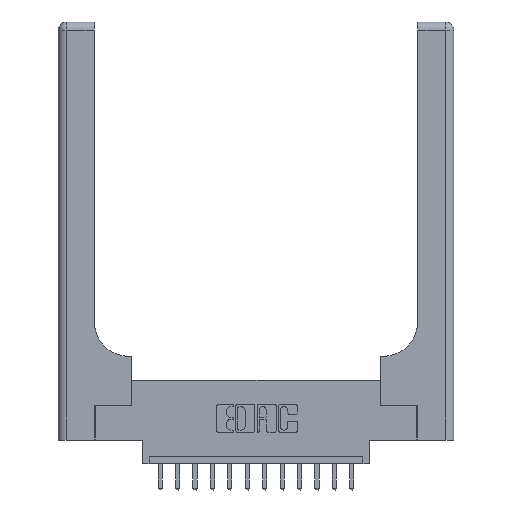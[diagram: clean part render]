
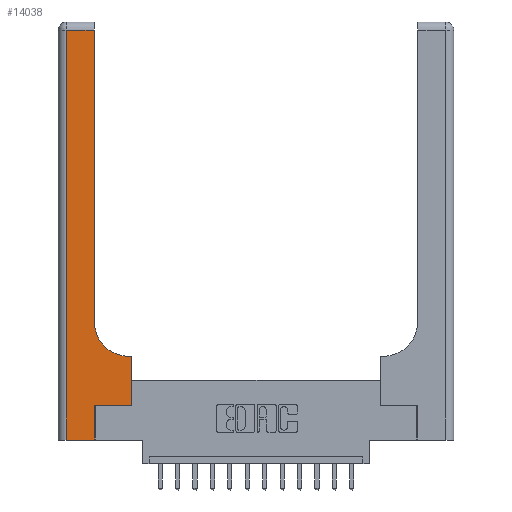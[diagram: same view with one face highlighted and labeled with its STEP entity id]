
A CAD part, top view. The second image highlights one B-rep face of the part: STEP entity #14038.
In plain terms, the highlighted planar face has unit normal (0, 0, 1).
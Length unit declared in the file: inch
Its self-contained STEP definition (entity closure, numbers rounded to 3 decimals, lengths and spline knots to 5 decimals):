
#672 = VERTEX_POINT ( 'NONE', #14484 ) ;
#717 = EDGE_LOOP ( 'NONE', ( #3443, #8007, #9765, #12176, #15172, #10499, #14028, #17084, #14723 ) ) ;
#1391 = CARTESIAN_POINT ( 'NONE',  ( 0.26, 2.94, 0.37 ) ) ;
#1451 = DIRECTION ( 'NONE',  ( 1., 0., 0. ) ) ;
#1673 = LINE ( 'NONE', #4305, #2613 ) ;
#2115 = AXIS2_PLACEMENT_3D ( 'NONE', #9466, #13533, #1451 ) ;
#2317 = CARTESIAN_POINT ( 'NONE',  ( 0.51, 0.6, 0.37 ) ) ;
#2613 = VECTOR ( 'NONE', #4220, 39.37008 ) ;
#2668 = EDGE_CURVE ( 'NONE', #10653, #672, #12846, .T. ) ;
#3202 = DIRECTION ( 'NONE',  ( 0., 1., 0. ) ) ;
#3443 = ORIENTED_EDGE ( 'NONE', *, *, #11669, .T. ) ;
#3545 = FACE_OUTER_BOUND ( 'NONE', #717, .T. ) ;
#3574 = VERTEX_POINT ( 'NONE', #16461 ) ;
#4220 = DIRECTION ( 'NONE',  ( -1., 0., 0. ) ) ;
#4304 = CARTESIAN_POINT ( 'NONE',  ( 0.265, 0.25, 0.37 ) ) ;
#4305 = CARTESIAN_POINT ( 'NONE',  ( 0.26, 0.6, 0.37 ) ) ;
#4487 = DIRECTION ( 'NONE',  ( 1., 0., 0. ) ) ;
#5463 = CARTESIAN_POINT ( 'NONE',  ( 0.528, 0.25, 0.37 ) ) ;
#5485 = CARTESIAN_POINT ( 'NONE',  ( 0.06, 3., 0.37 ) ) ;
#5790 = VECTOR ( 'NONE', #4487, 39.37008 ) ;
#6001 = CARTESIAN_POINT ( 'NONE',  ( 0., 2.94, 0.37 ) ) ;
#6024 = DIRECTION ( 'NONE',  ( 0., -1., 0. ) ) ;
#6605 = VECTOR ( 'NONE', #8547, 39.37008 ) ;
#6642 = CARTESIAN_POINT ( 'NONE',  ( 0.06, 0., 0.37 ) ) ;
#6781 = VERTEX_POINT ( 'NONE', #16806 ) ;
#6801 = LINE ( 'NONE', #5485, #17258 ) ;
#7393 = LINE ( 'NONE', #16512, #5790 ) ;
#7477 = AXIS2_PLACEMENT_3D ( 'NONE', #13007, #7615, #9206 ) ;
#7590 = EDGE_CURVE ( 'NONE', #9946, #16131, #15557, .T. ) ;
#7615 = DIRECTION ( 'NONE',  ( 0., 0., -1. ) ) ;
#8007 = ORIENTED_EDGE ( 'NONE', *, *, #11792, .T. ) ;
#8198 = VERTEX_POINT ( 'NONE', #10897 ) ;
#8436 = VERTEX_POINT ( 'NONE', #6642 ) ;
#8547 = DIRECTION ( 'NONE',  ( 0., 1., 0. ) ) ;
#8637 = VECTOR ( 'NONE', #3202, 39.37008 ) ;
#8883 = DIRECTION ( 'NONE',  ( -1., 0., 0. ) ) ;
#9206 = DIRECTION ( 'NONE',  ( -1., 0., 0. ) ) ;
#9246 = DIRECTION ( 'NONE',  ( 0., 1., 0. ) ) ;
#9452 = VERTEX_POINT ( 'NONE', #1391 ) ;
#9466 = CARTESIAN_POINT ( 'NONE',  ( 0.51, 0.85, 0.37 ) ) ;
#9696 = VECTOR ( 'NONE', #8883, 39.37008 ) ;
#9765 = ORIENTED_EDGE ( 'NONE', *, *, #15724, .T. ) ;
#9943 = LINE ( 'NONE', #16658, #6605 ) ;
#9946 = VERTEX_POINT ( 'NONE', #4304 ) ;
#10499 = ORIENTED_EDGE ( 'NONE', *, *, #7590, .T. ) ;
#10653 = VERTEX_POINT ( 'NONE', #2317 ) ;
#10897 = CARTESIAN_POINT ( 'NONE',  ( 0.06, 2.94, 0.37 ) ) ;
#11075 = EDGE_CURVE ( 'NONE', #6781, #10653, #1673, .T. ) ;
#11669 = EDGE_CURVE ( 'NONE', #672, #9452, #9943, .T. ) ;
#11792 = EDGE_CURVE ( 'NONE', #9452, #8198, #12693, .T. ) ;
#12176 = ORIENTED_EDGE ( 'NONE', *, *, #12475, .T. ) ;
#12475 = EDGE_CURVE ( 'NONE', #8436, #3574, #7393, .T. ) ;
#12693 = LINE ( 'NONE', #6001, #9696 ) ;
#12842 = CARTESIAN_POINT ( 'NONE',  ( 0.265, 0., 0.37 ) ) ;
#12846 = CIRCLE ( 'NONE', #2115, 0.25 ) ;
#13007 = CARTESIAN_POINT ( 'NONE',  ( 0., 3., 0.37 ) ) ;
#13533 = DIRECTION ( 'NONE',  ( 0., 0., -1. ) ) ;
#13568 = LINE ( 'NONE', #5463, #15363 ) ;
#13651 = CARTESIAN_POINT ( 'NONE',  ( 0.528, 0.25, 0.37 ) ) ;
#13905 = EDGE_CURVE ( 'NONE', #3574, #9946, #16550, .T. ) ;
#14028 = ORIENTED_EDGE ( 'NONE', *, *, #16123, .T. ) ;
#14038 = ADVANCED_FACE ( 'NONE', ( #3545 ), #17061, .F. ) ;
#14182 = CARTESIAN_POINT ( 'NONE',  ( 0.265, 0.25, 0.37 ) ) ;
#14239 = VECTOR ( 'NONE', #15477, 39.37008 ) ;
#14484 = CARTESIAN_POINT ( 'NONE',  ( 0.26, 0.85, 0.37 ) ) ;
#14723 = ORIENTED_EDGE ( 'NONE', *, *, #2668, .T. ) ;
#15172 = ORIENTED_EDGE ( 'NONE', *, *, #13905, .T. ) ;
#15363 = VECTOR ( 'NONE', #9246, 39.37008 ) ;
#15477 = DIRECTION ( 'NONE',  ( 1., 0., 0. ) ) ;
#15557 = LINE ( 'NONE', #14182, #14239 ) ;
#15724 = EDGE_CURVE ( 'NONE', #8198, #8436, #6801, .T. ) ;
#16123 = EDGE_CURVE ( 'NONE', #16131, #6781, #13568, .T. ) ;
#16131 = VERTEX_POINT ( 'NONE', #13651 ) ;
#16461 = CARTESIAN_POINT ( 'NONE',  ( 0.265, 0., 0.37 ) ) ;
#16512 = CARTESIAN_POINT ( 'NONE',  ( 0., 0., 0.37 ) ) ;
#16550 = LINE ( 'NONE', #12842, #8637 ) ;
#16658 = CARTESIAN_POINT ( 'NONE',  ( 0.26, 3., 0.37 ) ) ;
#16806 = CARTESIAN_POINT ( 'NONE',  ( 0.528, 0.6, 0.37 ) ) ;
#17061 = PLANE ( 'NONE',  #7477 ) ;
#17084 = ORIENTED_EDGE ( 'NONE', *, *, #11075, .T. ) ;
#17258 = VECTOR ( 'NONE', #6024, 39.37008 ) ;
